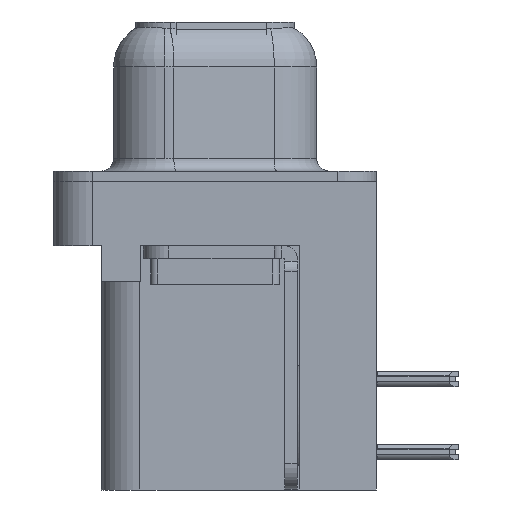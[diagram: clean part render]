
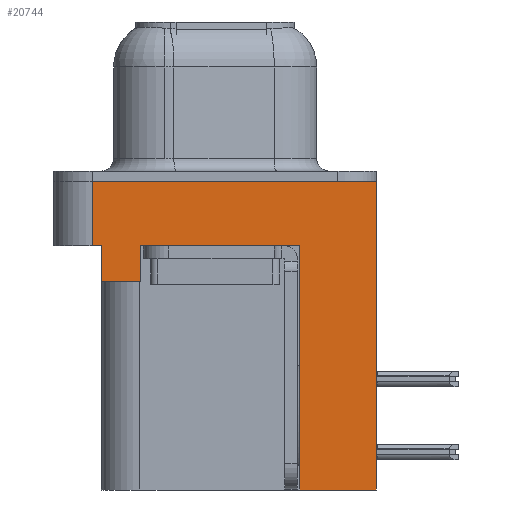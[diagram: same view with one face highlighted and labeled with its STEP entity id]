
A CAD part, left-side view. The second image highlights one B-rep face of the part: STEP entity #20744.
In plain terms, the highlighted planar face has unit normal (-1, 0, 0).
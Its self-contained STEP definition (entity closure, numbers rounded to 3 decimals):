
#171 = DIRECTION ( 'NONE',  ( -1., 0., 0. ) ) ;
#427 = EDGE_CURVE ( 'NONE', #7724, #29318, #12892, .T. ) ;
#693 = CARTESIAN_POINT ( 'NONE',  ( -2.91, 4.425, -2.5 ) ) ;
#1087 = CARTESIAN_POINT ( 'NONE',  ( -2.91, 4.775, 0. ) ) ;
#1102 = VECTOR ( 'NONE', #6624, 1000. ) ;
#1139 = VECTOR ( 'NONE', #27400, 1000. ) ;
#1521 = VECTOR ( 'NONE', #16180, 1000. ) ;
#3213 = PLANE ( 'NONE',  #16790 ) ;
#5795 = CARTESIAN_POINT ( 'NONE',  ( -2.91, 4.775, -2.5 ) ) ;
#5858 = EDGE_CURVE ( 'NONE', #25809, #32333, #16845, .T. ) ;
#6186 = VECTOR ( 'NONE', #22966, 1000. ) ;
#6418 = CARTESIAN_POINT ( 'NONE',  ( -2.91, 4.425, -3.9 ) ) ;
#6624 = DIRECTION ( 'NONE',  ( 0., 1., 0. ) ) ;
#6854 = VERTEX_POINT ( 'NONE', #18959 ) ;
#6873 = CARTESIAN_POINT ( 'NONE',  ( -2.91, 4.425, -3.9 ) ) ;
#7286 = EDGE_CURVE ( 'NONE', #21288, #7724, #33075, .T. ) ;
#7724 = VERTEX_POINT ( 'NONE', #13120 ) ;
#8790 = ORIENTED_EDGE ( 'NONE', *, *, #27769, .T. ) ;
#9145 = CARTESIAN_POINT ( 'NONE',  ( -2.91, -6.275, -2.5 ) ) ;
#9471 = CARTESIAN_POINT ( 'NONE',  ( -2.91, 2.895, -3.9 ) ) ;
#11085 = DIRECTION ( 'NONE',  ( 0., 0., 1. ) ) ;
#11595 = FACE_OUTER_BOUND ( 'NONE', #22295, .T. ) ;
#11928 = VECTOR ( 'NONE', #37769, 1000. ) ;
#11959 = DIRECTION ( 'NONE',  ( 0., 0., 1. ) ) ;
#12840 = CARTESIAN_POINT ( 'NONE',  ( -2.91, -6.275, 0. ) ) ;
#12892 = LINE ( 'NONE', #25473, #35454 ) ;
#13120 = CARTESIAN_POINT ( 'NONE',  ( -2.91, 2.895, -2.5 ) ) ;
#13925 = VECTOR ( 'NONE', #11959, 1000. ) ;
#14222 = ORIENTED_EDGE ( 'NONE', *, *, #19816, .F. ) ;
#14453 = ORIENTED_EDGE ( 'NONE', *, *, #7286, .T. ) ;
#14952 = CARTESIAN_POINT ( 'NONE',  ( -2.91, -6.275, -2.5 ) ) ;
#15074 = LINE ( 'NONE', #6418, #29805 ) ;
#15274 = CARTESIAN_POINT ( 'NONE',  ( -2.91, -6.275, -12. ) ) ;
#15610 = VECTOR ( 'NONE', #11085, 1000. ) ;
#15790 = DIRECTION ( 'NONE',  ( 0., 0., 1. ) ) ;
#15916 = LINE ( 'NONE', #6873, #1102 ) ;
#15976 = LINE ( 'NONE', #12840, #1139 ) ;
#16093 = CARTESIAN_POINT ( 'NONE',  ( -2.91, -3.295, -12. ) ) ;
#16180 = DIRECTION ( 'NONE',  ( 0., 0., 1. ) ) ;
#16376 = VERTEX_POINT ( 'NONE', #22585 ) ;
#16715 = CARTESIAN_POINT ( 'NONE',  ( -2.91, -3.295, -12. ) ) ;
#16790 = AXIS2_PLACEMENT_3D ( 'NONE', #14952, #171, #18043 ) ;
#16845 = LINE ( 'NONE', #28169, #1521 ) ;
#17335 = VERTEX_POINT ( 'NONE', #16093 ) ;
#17928 = ORIENTED_EDGE ( 'NONE', *, *, #29968, .F. ) ;
#18043 = DIRECTION ( 'NONE',  ( 0., 0., 1. ) ) ;
#18959 = CARTESIAN_POINT ( 'NONE',  ( -2.91, 4.425, -3.9 ) ) ;
#19816 = EDGE_CURVE ( 'NONE', #16376, #34410, #35128, .T. ) ;
#20035 = VERTEX_POINT ( 'NONE', #693 ) ;
#20418 = ORIENTED_EDGE ( 'NONE', *, *, #34600, .F. ) ;
#20744 = ADVANCED_FACE ( 'NONE', ( #11595 ), #3213, .T. ) ;
#21288 = VERTEX_POINT ( 'NONE', #9471 ) ;
#22295 = EDGE_LOOP ( 'NONE', ( #30575, #14222, #8790, #32280, #23226, #14453, #22573, #20418, #17928, #32090 ) ) ;
#22573 = ORIENTED_EDGE ( 'NONE', *, *, #427, .T. ) ;
#22585 = CARTESIAN_POINT ( 'NONE',  ( -2.91, 4.775, -2.5 ) ) ;
#22753 = EDGE_CURVE ( 'NONE', #21288, #6854, #15916, .T. ) ;
#22966 = DIRECTION ( 'NONE',  ( 0., 1., 0. ) ) ;
#23164 = CARTESIAN_POINT ( 'NONE',  ( -2.91, -3.295, -12. ) ) ;
#23226 = ORIENTED_EDGE ( 'NONE', *, *, #22753, .F. ) ;
#23473 = LINE ( 'NONE', #23164, #15610 ) ;
#25473 = CARTESIAN_POINT ( 'NONE',  ( -2.91, -6.275, -2.5 ) ) ;
#25596 = DIRECTION ( 'NONE',  ( 0., -1., 0. ) ) ;
#25809 = VERTEX_POINT ( 'NONE', #15274 ) ;
#25822 = EDGE_CURVE ( 'NONE', #34410, #32333, #15976, .T. ) ;
#25994 = LINE ( 'NONE', #16715, #6186 ) ;
#27400 = DIRECTION ( 'NONE',  ( 0., -1., 0. ) ) ;
#27769 = EDGE_CURVE ( 'NONE', #16376, #20035, #37677, .T. ) ;
#28094 = EDGE_CURVE ( 'NONE', #6854, #20035, #15074, .T. ) ;
#28122 = CARTESIAN_POINT ( 'NONE',  ( -2.91, 2.895, -3.9 ) ) ;
#28169 = CARTESIAN_POINT ( 'NONE',  ( -2.91, -6.275, -2.5 ) ) ;
#29318 = VERTEX_POINT ( 'NONE', #29481 ) ;
#29481 = CARTESIAN_POINT ( 'NONE',  ( -2.91, -3.295, -2.5 ) ) ;
#29805 = VECTOR ( 'NONE', #15790, 1000. ) ;
#29968 = EDGE_CURVE ( 'NONE', #25809, #17335, #25994, .T. ) ;
#29992 = DIRECTION ( 'NONE',  ( 0., -1., 0. ) ) ;
#30575 = ORIENTED_EDGE ( 'NONE', *, *, #25822, .F. ) ;
#32090 = ORIENTED_EDGE ( 'NONE', *, *, #5858, .T. ) ;
#32280 = ORIENTED_EDGE ( 'NONE', *, *, #28094, .F. ) ;
#32333 = VERTEX_POINT ( 'NONE', #33711 ) ;
#33075 = LINE ( 'NONE', #28122, #11928 ) ;
#33711 = CARTESIAN_POINT ( 'NONE',  ( -2.91, -6.275, 0. ) ) ;
#34410 = VERTEX_POINT ( 'NONE', #1087 ) ;
#34600 = EDGE_CURVE ( 'NONE', #17335, #29318, #23473, .T. ) ;
#35128 = LINE ( 'NONE', #5795, #13925 ) ;
#35454 = VECTOR ( 'NONE', #25596, 1000. ) ;
#35810 = VECTOR ( 'NONE', #29992, 1000. ) ;
#37677 = LINE ( 'NONE', #9145, #35810 ) ;
#37769 = DIRECTION ( 'NONE',  ( 0., 0., 1. ) ) ;
